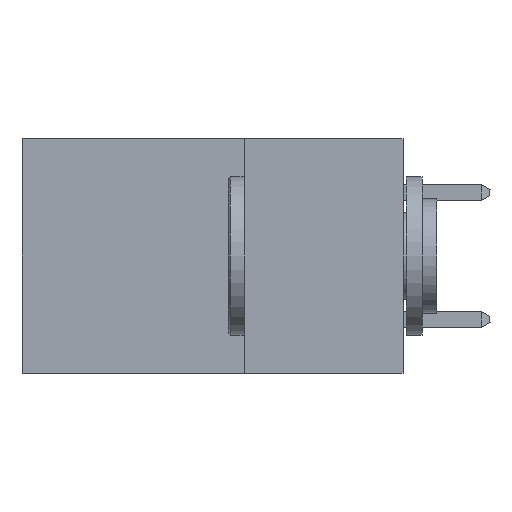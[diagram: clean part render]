
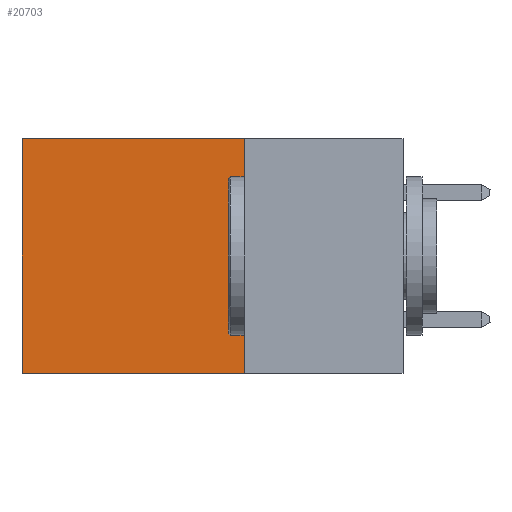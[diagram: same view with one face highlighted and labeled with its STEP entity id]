
A CAD part, left-side view. The second image highlights one B-rep face of the part: STEP entity #20703.
In plain terms, the highlighted planar face has unit normal (-1, 0, 0).
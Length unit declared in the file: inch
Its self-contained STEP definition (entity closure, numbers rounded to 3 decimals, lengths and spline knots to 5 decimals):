
#232 = VECTOR ( 'NONE', #20732, 39.37008 ) ;
#1290 = DIRECTION ( 'NONE',  ( 1., 0., 0. ) ) ;
#1476 = AXIS2_PLACEMENT_3D ( 'NONE', #20948, #1290, #12841 ) ;
#1889 = VERTEX_POINT ( 'NONE', #11730 ) ;
#3175 = CARTESIAN_POINT ( 'NONE',  ( 0.2875, 0.6, -0.37 ) ) ;
#3926 = EDGE_CURVE ( 'NONE', #1889, #15970, #13908, .T. ) ;
#4008 = ORIENTED_EDGE ( 'NONE', *, *, #20697, .F. ) ;
#5201 = LINE ( 'NONE', #15835, #232 ) ;
#5450 = EDGE_LOOP ( 'NONE', ( #9776, #5880, #4008, #18793 ) ) ;
#5880 = ORIENTED_EDGE ( 'NONE', *, *, #13617, .F. ) ;
#6394 = LINE ( 'NONE', #16053, #17957 ) ;
#9072 = VECTOR ( 'NONE', #10268, 39.37008 ) ;
#9776 = ORIENTED_EDGE ( 'NONE', *, *, #3926, .T. ) ;
#9792 = FACE_OUTER_BOUND ( 'NONE', #5450, .T. ) ;
#10268 = DIRECTION ( 'NONE',  ( 0., 0., -1. ) ) ;
#11730 = CARTESIAN_POINT ( 'NONE',  ( 0.2875, 0.6, 0. ) ) ;
#12153 = CARTESIAN_POINT ( 'NONE',  ( 0.2875, 0.25, -0.37 ) ) ;
#12479 = CARTESIAN_POINT ( 'NONE',  ( 0.2875, 0.6, 0. ) ) ;
#12841 = DIRECTION ( 'NONE',  ( 0., 0., -1. ) ) ;
#13617 = EDGE_CURVE ( 'NONE', #19793, #15970, #5201, .T. ) ;
#13908 = LINE ( 'NONE', #12479, #9072 ) ;
#15031 = VECTOR ( 'NONE', #16161, 39.37008 ) ;
#15543 = LINE ( 'NONE', #20979, #15031 ) ;
#15835 = CARTESIAN_POINT ( 'NONE',  ( 0.2875, 0.25, -0.37 ) ) ;
#15970 = VERTEX_POINT ( 'NONE', #3175 ) ;
#16053 = CARTESIAN_POINT ( 'NONE',  ( 0.2875, 0.25, 0. ) ) ;
#16161 = DIRECTION ( 'NONE',  ( 0., 1., 0. ) ) ;
#16837 = EDGE_CURVE ( 'NONE', #18512, #1889, #15543, .T. ) ;
#17719 = DIRECTION ( 'NONE',  ( 0., 0., -1. ) ) ;
#17957 = VECTOR ( 'NONE', #17719, 39.37008 ) ;
#18512 = VERTEX_POINT ( 'NONE', #20552 ) ;
#18793 = ORIENTED_EDGE ( 'NONE', *, *, #16837, .T. ) ;
#19332 = PLANE ( 'NONE',  #1476 ) ;
#19793 = VERTEX_POINT ( 'NONE', #12153 ) ;
#20552 = CARTESIAN_POINT ( 'NONE',  ( 0.2875, 0.25, 0. ) ) ;
#20697 = EDGE_CURVE ( 'NONE', #18512, #19793, #6394, .T. ) ;
#20703 = ADVANCED_FACE ( 'NONE', ( #9792 ), #19332, .F. ) ;
#20732 = DIRECTION ( 'NONE',  ( 0., 1., 0. ) ) ;
#20948 = CARTESIAN_POINT ( 'NONE',  ( 0.2875, 0.25, 0. ) ) ;
#20979 = CARTESIAN_POINT ( 'NONE',  ( 0.2875, 0.25, 0. ) ) ;
